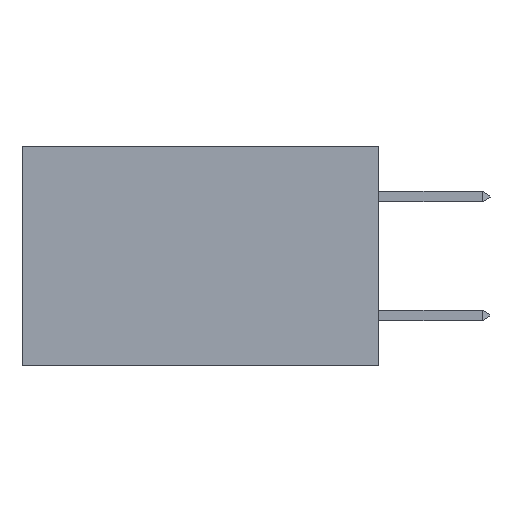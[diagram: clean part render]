
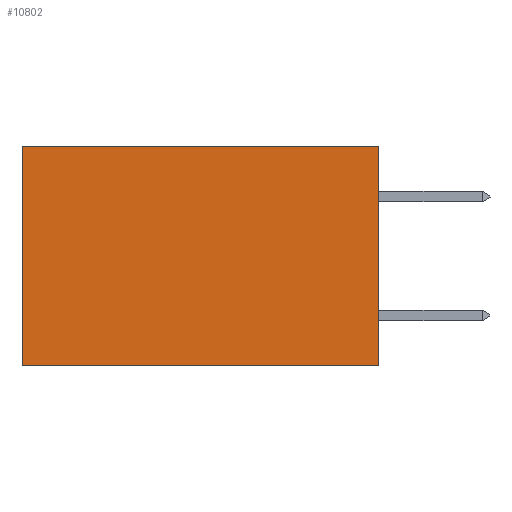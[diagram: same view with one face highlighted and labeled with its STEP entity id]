
A CAD part, left-side view. The second image highlights one B-rep face of the part: STEP entity #10802.
In plain terms, the highlighted planar face has unit normal (-1, 0, 0).
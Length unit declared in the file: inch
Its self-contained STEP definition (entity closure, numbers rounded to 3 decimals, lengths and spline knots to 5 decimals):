
#82 = ORIENTED_EDGE ( 'NONE', *, *, #16691, .F. ) ;
#420 = CARTESIAN_POINT ( 'NONE',  ( 0.298, 0.6, 0. ) ) ;
#707 = CARTESIAN_POINT ( 'NONE',  ( 0.298, 0., 0. ) ) ;
#1071 = EDGE_LOOP ( 'NONE', ( #14683, #82, #10697, #13996 ) ) ;
#2421 = CARTESIAN_POINT ( 'NONE',  ( 0.298, 0., -0.37 ) ) ;
#2659 = DIRECTION ( 'NONE',  ( 0., 0., -1. ) ) ;
#2822 = CARTESIAN_POINT ( 'NONE',  ( 0.298, 0., 0. ) ) ;
#2871 = VECTOR ( 'NONE', #12239, 39.37008 ) ;
#3293 = VERTEX_POINT ( 'NONE', #10254 ) ;
#3690 = EDGE_CURVE ( 'NONE', #5969, #10675, #8108, .T. ) ;
#3736 = DIRECTION ( 'NONE',  ( 0., 0., -1. ) ) ;
#3815 = LINE ( 'NONE', #707, #7702 ) ;
#4453 = CARTESIAN_POINT ( 'NONE',  ( 0.298, 0., 0. ) ) ;
#4463 = EDGE_CURVE ( 'NONE', #17907, #5969, #19497, .T. ) ;
#5477 = AXIS2_PLACEMENT_3D ( 'NONE', #2822, #11333, #6741 ) ;
#5969 = VERTEX_POINT ( 'NONE', #15847 ) ;
#6217 = PLANE ( 'NONE',  #5477 ) ;
#6741 = DIRECTION ( 'NONE',  ( 0., 0., -1. ) ) ;
#7318 = VECTOR ( 'NONE', #11203, 39.37008 ) ;
#7702 = VECTOR ( 'NONE', #2659, 39.37008 ) ;
#7895 = CARTESIAN_POINT ( 'NONE',  ( 0.298, 0., 0. ) ) ;
#8108 = LINE ( 'NONE', #420, #18237 ) ;
#10176 = EDGE_CURVE ( 'NONE', #17907, #3293, #3815, .T. ) ;
#10254 = CARTESIAN_POINT ( 'NONE',  ( 0.298, 0., -0.37 ) ) ;
#10675 = VERTEX_POINT ( 'NONE', #15630 ) ;
#10697 = ORIENTED_EDGE ( 'NONE', *, *, #10176, .F. ) ;
#10802 = ADVANCED_FACE ( 'NONE', ( #16493 ), #6217, .F. ) ;
#11203 = DIRECTION ( 'NONE',  ( 0., 1., 0. ) ) ;
#11333 = DIRECTION ( 'NONE',  ( 1., 0., 0. ) ) ;
#11904 = LINE ( 'NONE', #2421, #2871 ) ;
#12239 = DIRECTION ( 'NONE',  ( 0., 1., 0. ) ) ;
#13996 = ORIENTED_EDGE ( 'NONE', *, *, #4463, .T. ) ;
#14683 = ORIENTED_EDGE ( 'NONE', *, *, #3690, .T. ) ;
#15630 = CARTESIAN_POINT ( 'NONE',  ( 0.298, 0.6, -0.37 ) ) ;
#15847 = CARTESIAN_POINT ( 'NONE',  ( 0.298, 0.6, 0. ) ) ;
#16493 = FACE_OUTER_BOUND ( 'NONE', #1071, .T. ) ;
#16691 = EDGE_CURVE ( 'NONE', #3293, #10675, #11904, .T. ) ;
#17907 = VERTEX_POINT ( 'NONE', #4453 ) ;
#18237 = VECTOR ( 'NONE', #3736, 39.37008 ) ;
#19497 = LINE ( 'NONE', #7895, #7318 ) ;
